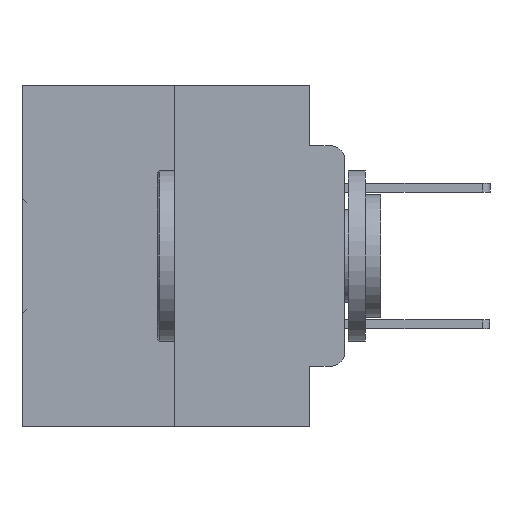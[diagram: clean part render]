
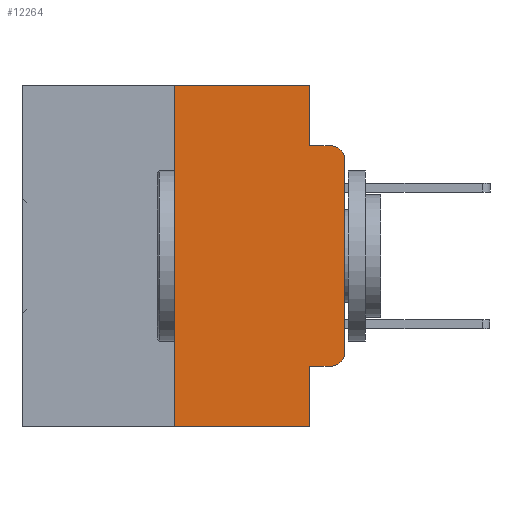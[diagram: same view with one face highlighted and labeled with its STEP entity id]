
A CAD part, left-side view. The second image highlights one B-rep face of the part: STEP entity #12264.
In plain terms, the highlighted planar face has unit normal (-1, 0, 0).
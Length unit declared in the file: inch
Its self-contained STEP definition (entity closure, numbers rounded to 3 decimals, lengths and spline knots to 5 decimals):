
#870 = EDGE_CURVE ( 'NONE', #7452, #5831, #4810, .T. ) ;
#1363 = VECTOR ( 'NONE', #3399, 39.37008 ) ;
#1515 = VERTEX_POINT ( 'NONE', #2618 ) ;
#1807 = AXIS2_PLACEMENT_3D ( 'NONE', #9380, #28322, #12101 ) ;
#1921 = VECTOR ( 'NONE', #30393, 39.37008 ) ;
#2266 = DIRECTION ( 'NONE',  ( 0., -1., 0. ) ) ;
#2500 = VECTOR ( 'NONE', #5595, 39.37008 ) ;
#2618 = CARTESIAN_POINT ( 'NONE',  ( 0., 0., -0.3915 ) ) ;
#2759 = LINE ( 'NONE', #22246, #1921 ) ;
#3332 = CARTESIAN_POINT ( 'NONE',  ( 0., 0., -0.1085 ) ) ;
#3399 = DIRECTION ( 'NONE',  ( 0., -1., 0. ) ) ;
#3497 = CARTESIAN_POINT ( 'NONE',  ( 0., 0.473, 0. ) ) ;
#3757 = CARTESIAN_POINT ( 'NONE',  ( 0., 0.02, -0.3915 ) ) ;
#4810 = LINE ( 'NONE', #27064, #24779 ) ;
#5063 = VECTOR ( 'NONE', #22469, 39.37008 ) ;
#5104 = VERTEX_POINT ( 'NONE', #26913 ) ;
#5370 = CARTESIAN_POINT ( 'NONE',  ( 0., 0., 0. ) ) ;
#5595 = DIRECTION ( 'NONE',  ( 0., 0., -1. ) ) ;
#5831 = VERTEX_POINT ( 'NONE', #10886 ) ;
#5950 = EDGE_CURVE ( 'NONE', #5831, #27969, #2759, .T. ) ;
#5984 = ORIENTED_EDGE ( 'NONE', *, *, #12277, .T. ) ;
#6132 = CARTESIAN_POINT ( 'NONE',  ( 0., 0.473, -0.5 ) ) ;
#6417 = EDGE_CURVE ( 'NONE', #1515, #11690, #23511, .T. ) ;
#6503 = DIRECTION ( 'NONE',  ( 0., 0., -1. ) ) ;
#7161 = CIRCLE ( 'NONE', #12620, 0.02 ) ;
#7254 = EDGE_CURVE ( 'NONE', #11690, #27969, #24307, .T. ) ;
#7452 = VERTEX_POINT ( 'NONE', #10197 ) ;
#8468 = ORIENTED_EDGE ( 'NONE', *, *, #6417, .T. ) ;
#8555 = LINE ( 'NONE', #6132, #1363 ) ;
#8723 = PLANE ( 'NONE',  #32669 ) ;
#8962 = CARTESIAN_POINT ( 'NONE',  ( 0., 0.051, -0.5 ) ) ;
#9033 = EDGE_CURVE ( 'NONE', #24593, #7452, #27556, .T. ) ;
#9380 = CARTESIAN_POINT ( 'NONE',  ( 0., 0.02, -0.1085 ) ) ;
#9545 = EDGE_CURVE ( 'NONE', #34281, #29953, #9703, .T. ) ;
#9703 = LINE ( 'NONE', #32510, #2500 ) ;
#9974 = CARTESIAN_POINT ( 'NONE',  ( 0., 0.25, 0. ) ) ;
#10197 = CARTESIAN_POINT ( 'NONE',  ( 0., 0.051, 0. ) ) ;
#10201 = ORIENTED_EDGE ( 'NONE', *, *, #5950, .F. ) ;
#10841 = DIRECTION ( 'NONE',  ( 0., 0., 1. ) ) ;
#10886 = CARTESIAN_POINT ( 'NONE',  ( 0., 0.051, -0.0885 ) ) ;
#11083 = DIRECTION ( 'NONE',  ( 0., 0., -1. ) ) ;
#11607 = CARTESIAN_POINT ( 'NONE',  ( 0., 0.25, 0. ) ) ;
#11690 = VERTEX_POINT ( 'NONE', #3332 ) ;
#12101 = DIRECTION ( 'NONE',  ( 0., 0., -1. ) ) ;
#12264 = ADVANCED_FACE ( 'NONE', ( #15787 ), #8723, .F. ) ;
#12277 = EDGE_CURVE ( 'NONE', #5104, #29953, #8555, .T. ) ;
#12620 = AXIS2_PLACEMENT_3D ( 'NONE', #3757, #22735, #6503 ) ;
#13173 = ORIENTED_EDGE ( 'NONE', *, *, #14645, .T. ) ;
#13611 = ORIENTED_EDGE ( 'NONE', *, *, #870, .F. ) ;
#14208 = DIRECTION ( 'NONE',  ( 0., 0., -1. ) ) ;
#14645 = EDGE_CURVE ( 'NONE', #25036, #1515, #7161, .T. ) ;
#15787 = FACE_OUTER_BOUND ( 'NONE', #29594, .T. ) ;
#16210 = CARTESIAN_POINT ( 'NONE',  ( 0., 0.02, -0.4115 ) ) ;
#16537 = ORIENTED_EDGE ( 'NONE', *, *, #7254, .T. ) ;
#17203 = EDGE_CURVE ( 'NONE', #5104, #24593, #22106, .T. ) ;
#20076 = CARTESIAN_POINT ( 'NONE',  ( 0., 0.02, -0.0885 ) ) ;
#21219 = CARTESIAN_POINT ( 'NONE',  ( 0., 0.051, -0.4115 ) ) ;
#21816 = VECTOR ( 'NONE', #10841, 39.37008 ) ;
#21913 = CARTESIAN_POINT ( 'NONE',  ( 0., 0.051, -0.4115 ) ) ;
#22106 = LINE ( 'NONE', #9974, #26747 ) ;
#22246 = CARTESIAN_POINT ( 'NONE',  ( 0., 0.051, -0.0885 ) ) ;
#22248 = CARTESIAN_POINT ( 'NONE',  ( 0., 0.473, 0. ) ) ;
#22469 = DIRECTION ( 'NONE',  ( 0., -1., 0. ) ) ;
#22498 = ORIENTED_EDGE ( 'NONE', *, *, #9033, .F. ) ;
#22735 = DIRECTION ( 'NONE',  ( -1., 0., 0. ) ) ;
#23511 = LINE ( 'NONE', #5370, #21816 ) ;
#23797 = ORIENTED_EDGE ( 'NONE', *, *, #9545, .F. ) ;
#24217 = ORIENTED_EDGE ( 'NONE', *, *, #17203, .F. ) ;
#24307 = CIRCLE ( 'NONE', #1807, 0.02 ) ;
#24593 = VERTEX_POINT ( 'NONE', #11607 ) ;
#24661 = ORIENTED_EDGE ( 'NONE', *, *, #32979, .T. ) ;
#24779 = VECTOR ( 'NONE', #11083, 39.37008 ) ;
#25036 = VERTEX_POINT ( 'NONE', #16210 ) ;
#26747 = VECTOR ( 'NONE', #28921, 39.37008 ) ;
#26913 = CARTESIAN_POINT ( 'NONE',  ( 0., 0.25, -0.5 ) ) ;
#26934 = VECTOR ( 'NONE', #2266, 39.37008 ) ;
#27064 = CARTESIAN_POINT ( 'NONE',  ( 0., 0.051, 0. ) ) ;
#27556 = LINE ( 'NONE', #3497, #5063 ) ;
#27969 = VERTEX_POINT ( 'NONE', #20076 ) ;
#28322 = DIRECTION ( 'NONE',  ( -1., 0., 0. ) ) ;
#28921 = DIRECTION ( 'NONE',  ( 0., 0., 1. ) ) ;
#29594 = EDGE_LOOP ( 'NONE', ( #8468, #16537, #10201, #13611, #22498, #24217, #5984, #23797, #24661, #13173 ) ) ;
#29953 = VERTEX_POINT ( 'NONE', #8962 ) ;
#30393 = DIRECTION ( 'NONE',  ( 0., -1., 0. ) ) ;
#32510 = CARTESIAN_POINT ( 'NONE',  ( 0., 0.051, 0. ) ) ;
#32669 = AXIS2_PLACEMENT_3D ( 'NONE', #22248, #32905, #14208 ) ;
#32905 = DIRECTION ( 'NONE',  ( 1., 0., 0. ) ) ;
#32979 = EDGE_CURVE ( 'NONE', #34281, #25036, #34808, .T. ) ;
#34281 = VERTEX_POINT ( 'NONE', #21913 ) ;
#34808 = LINE ( 'NONE', #21219, #26934 ) ;
